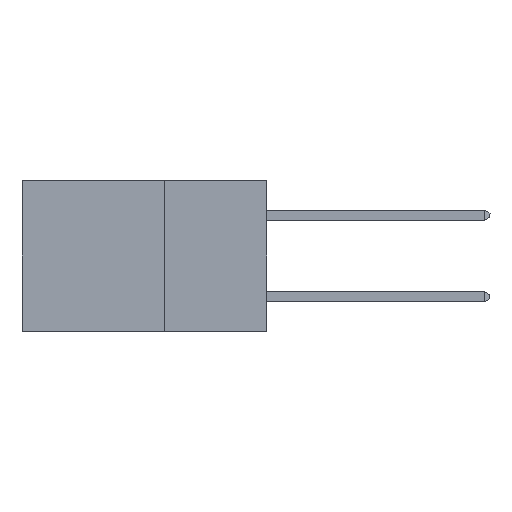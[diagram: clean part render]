
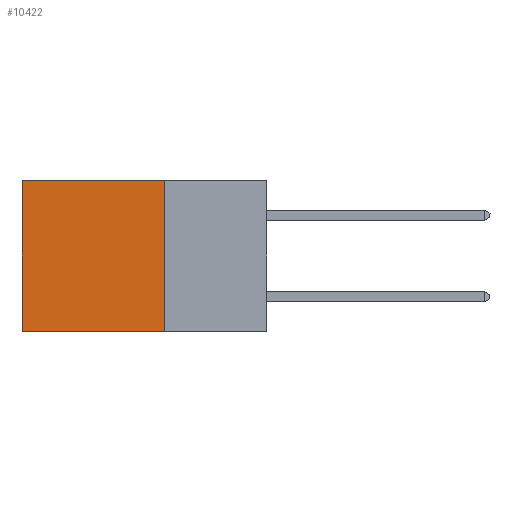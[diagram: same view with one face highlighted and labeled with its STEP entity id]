
A CAD part, left-side view. The second image highlights one B-rep face of the part: STEP entity #10422.
In plain terms, the highlighted planar face has unit normal (-1, 0, 0).
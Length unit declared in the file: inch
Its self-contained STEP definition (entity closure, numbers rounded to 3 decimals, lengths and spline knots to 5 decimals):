
#422 = CARTESIAN_POINT ( 'NONE',  ( 0.2875, 0.25, 0. ) ) ;
#869 = LINE ( 'NONE', #422, #3263 ) ;
#1604 = DIRECTION ( 'NONE',  ( 0., 1., 0. ) ) ;
#2287 = VECTOR ( 'NONE', #1604, 39.37008 ) ;
#2790 = EDGE_LOOP ( 'NONE', ( #5873, #11533, #7986, #10907 ) ) ;
#3263 = VECTOR ( 'NONE', #5600, 39.37008 ) ;
#3532 = CARTESIAN_POINT ( 'NONE',  ( 0.2875, 0.6, -0.37 ) ) ;
#3577 = EDGE_CURVE ( 'NONE', #5614, #10593, #10512, .T. ) ;
#4176 = EDGE_CURVE ( 'NONE', #5614, #9213, #869, .T. ) ;
#4346 = CARTESIAN_POINT ( 'NONE',  ( 0.2875, 0.25, -0.37 ) ) ;
#4835 = FACE_OUTER_BOUND ( 'NONE', #2790, .T. ) ;
#5537 = LINE ( 'NONE', #4346, #7990 ) ;
#5600 = DIRECTION ( 'NONE',  ( 0., 0., -1. ) ) ;
#5614 = VERTEX_POINT ( 'NONE', #12734 ) ;
#5873 = ORIENTED_EDGE ( 'NONE', *, *, #10693, .T. ) ;
#6450 = DIRECTION ( 'NONE',  ( 0., 0., -1. ) ) ;
#7464 = AXIS2_PLACEMENT_3D ( 'NONE', #10495, #12572, #6450 ) ;
#7986 = ORIENTED_EDGE ( 'NONE', *, *, #4176, .F. ) ;
#7990 = VECTOR ( 'NONE', #12581, 39.37008 ) ;
#8012 = EDGE_CURVE ( 'NONE', #9213, #11860, #5537, .T. ) ;
#8811 = DIRECTION ( 'NONE',  ( 0., 0., -1. ) ) ;
#8821 = CARTESIAN_POINT ( 'NONE',  ( 0.2875, 0.25, 0. ) ) ;
#8850 = CARTESIAN_POINT ( 'NONE',  ( 0.2875, 0.6, 0. ) ) ;
#9196 = LINE ( 'NONE', #8850, #11926 ) ;
#9213 = VERTEX_POINT ( 'NONE', #11715 ) ;
#10422 = ADVANCED_FACE ( 'NONE', ( #4835 ), #12531, .F. ) ;
#10495 = CARTESIAN_POINT ( 'NONE',  ( 0.2875, 0.25, 0. ) ) ;
#10512 = LINE ( 'NONE', #8821, #2287 ) ;
#10593 = VERTEX_POINT ( 'NONE', #12746 ) ;
#10693 = EDGE_CURVE ( 'NONE', #10593, #11860, #9196, .T. ) ;
#10907 = ORIENTED_EDGE ( 'NONE', *, *, #3577, .T. ) ;
#11533 = ORIENTED_EDGE ( 'NONE', *, *, #8012, .F. ) ;
#11715 = CARTESIAN_POINT ( 'NONE',  ( 0.2875, 0.25, -0.37 ) ) ;
#11860 = VERTEX_POINT ( 'NONE', #3532 ) ;
#11926 = VECTOR ( 'NONE', #8811, 39.37008 ) ;
#12531 = PLANE ( 'NONE',  #7464 ) ;
#12572 = DIRECTION ( 'NONE',  ( 1., 0., 0. ) ) ;
#12581 = DIRECTION ( 'NONE',  ( 0., 1., 0. ) ) ;
#12734 = CARTESIAN_POINT ( 'NONE',  ( 0.2875, 0.25, 0. ) ) ;
#12746 = CARTESIAN_POINT ( 'NONE',  ( 0.2875, 0.6, 0. ) ) ;
